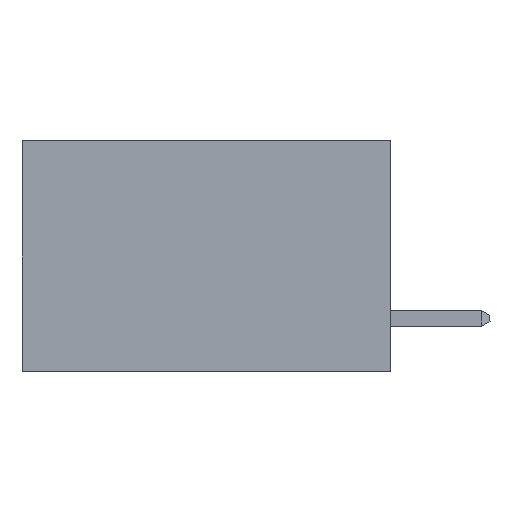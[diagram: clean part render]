
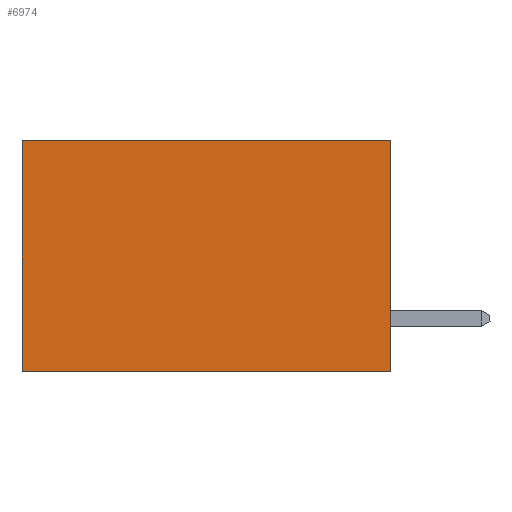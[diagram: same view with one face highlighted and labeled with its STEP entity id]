
A CAD part, left-side view. The second image highlights one B-rep face of the part: STEP entity #6974.
In plain terms, the highlighted planar face has unit normal (-1, 0, 0).
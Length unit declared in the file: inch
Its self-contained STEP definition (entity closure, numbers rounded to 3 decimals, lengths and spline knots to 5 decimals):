
#477 = CARTESIAN_POINT ( 'NONE',  ( 0.277, 0.59, -0.37 ) ) ;
#722 = FACE_OUTER_BOUND ( 'NONE', #9144, .T. ) ;
#817 = ORIENTED_EDGE ( 'NONE', *, *, #10413, .F. ) ;
#980 = DIRECTION ( 'NONE',  ( 0., 1., 0. ) ) ;
#1083 = DIRECTION ( 'NONE',  ( 0., 0., -1. ) ) ;
#1098 = ORIENTED_EDGE ( 'NONE', *, *, #3354, .T. ) ;
#1252 = CARTESIAN_POINT ( 'NONE',  ( 0.277, 0.59, -0.37 ) ) ;
#1831 = EDGE_CURVE ( 'NONE', #7220, #2492, #7174, .T. ) ;
#2211 = CARTESIAN_POINT ( 'NONE',  ( 0.277, 0., -0.37 ) ) ;
#2416 = CARTESIAN_POINT ( 'NONE',  ( 0.277, 0., -0.37 ) ) ;
#2492 = VERTEX_POINT ( 'NONE', #477 ) ;
#2592 = LINE ( 'NONE', #2730, #4433 ) ;
#2730 = CARTESIAN_POINT ( 'NONE',  ( 0.277, 0., -0.37 ) ) ;
#3354 = EDGE_CURVE ( 'NONE', #4059, #7220, #3447, .T. ) ;
#3447 = LINE ( 'NONE', #11045, #7813 ) ;
#3865 = PLANE ( 'NONE',  #9744 ) ;
#4059 = VERTEX_POINT ( 'NONE', #7409 ) ;
#4403 = VECTOR ( 'NONE', #1083, 39.37008 ) ;
#4433 = VECTOR ( 'NONE', #980, 39.37008 ) ;
#4765 = CARTESIAN_POINT ( 'NONE',  ( 0.277, 0., -0.37 ) ) ;
#4775 = DIRECTION ( 'NONE',  ( 0., 0., -1. ) ) ;
#5100 = VERTEX_POINT ( 'NONE', #2211 ) ;
#5320 = EDGE_CURVE ( 'NONE', #4059, #5100, #6705, .T. ) ;
#5620 = DIRECTION ( 'NONE',  ( 0., 0., -1. ) ) ;
#6705 = LINE ( 'NONE', #2416, #4403 ) ;
#6974 = ADVANCED_FACE ( 'NONE', ( #722 ), #3865, .F. ) ;
#7174 = LINE ( 'NONE', #1252, #9471 ) ;
#7220 = VERTEX_POINT ( 'NONE', #10261 ) ;
#7409 = CARTESIAN_POINT ( 'NONE',  ( 0.277, 0., 0. ) ) ;
#7588 = ORIENTED_EDGE ( 'NONE', *, *, #1831, .T. ) ;
#7813 = VECTOR ( 'NONE', #11034, 39.37008 ) ;
#9144 = EDGE_LOOP ( 'NONE', ( #7588, #817, #10122, #1098 ) ) ;
#9471 = VECTOR ( 'NONE', #4775, 39.37008 ) ;
#9744 = AXIS2_PLACEMENT_3D ( 'NONE', #4765, #10760, #5620 ) ;
#10122 = ORIENTED_EDGE ( 'NONE', *, *, #5320, .F. ) ;
#10261 = CARTESIAN_POINT ( 'NONE',  ( 0.277, 0.59, 0. ) ) ;
#10413 = EDGE_CURVE ( 'NONE', #5100, #2492, #2592, .T. ) ;
#10760 = DIRECTION ( 'NONE',  ( 1., 0., 0. ) ) ;
#11034 = DIRECTION ( 'NONE',  ( 0., 1., 0. ) ) ;
#11045 = CARTESIAN_POINT ( 'NONE',  ( 0.277, 0., 0. ) ) ;
